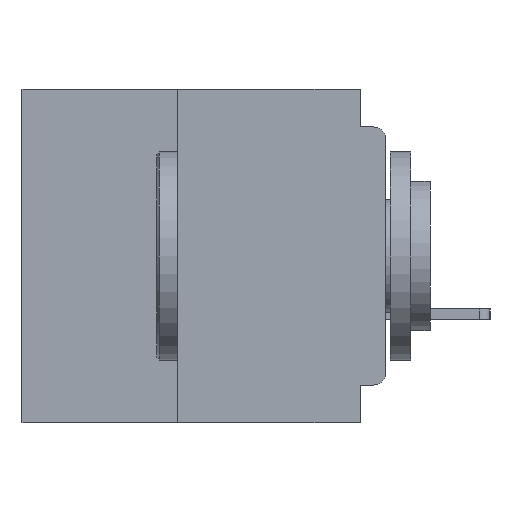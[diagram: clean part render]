
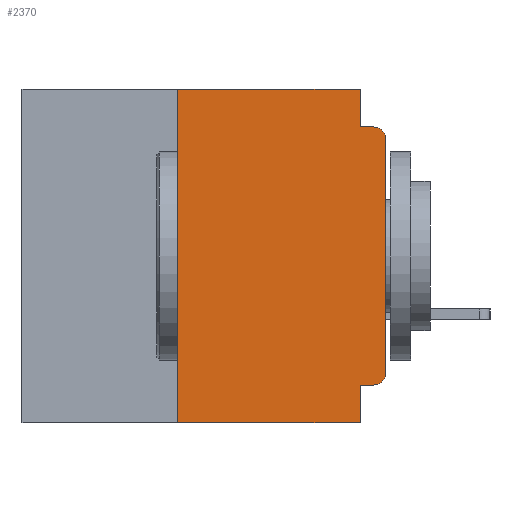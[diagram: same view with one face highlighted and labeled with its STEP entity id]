
A CAD part, left-side view. The second image highlights one B-rep face of the part: STEP entity #2370.
In plain terms, the highlighted planar face has unit normal (-1, 0, 0).
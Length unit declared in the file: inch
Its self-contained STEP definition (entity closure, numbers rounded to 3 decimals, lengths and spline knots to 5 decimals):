
#1368 = VECTOR ( 'NONE', #28148, 39.37008 ) ;
#1810 = VERTEX_POINT ( 'NONE', #24795 ) ;
#2370 = ADVANCED_FACE ( 'NONE', ( #47986 ), #18815, .F. ) ;
#2901 = EDGE_CURVE ( 'NONE', #58444, #57417, #28185, .T. ) ;
#2973 = LINE ( 'NONE', #21634, #39948 ) ;
#4911 = EDGE_CURVE ( 'NONE', #58444, #41368, #53182, .T. ) ;
#6284 = DIRECTION ( 'NONE',  ( 0., 0., -1. ) ) ;
#6732 = DIRECTION ( 'NONE',  ( 0., 0., -1. ) ) ;
#7279 = ORIENTED_EDGE ( 'NONE', *, *, #32563, .F. ) ;
#7483 = VECTOR ( 'NONE', #6284, 39.37008 ) ;
#8209 = CARTESIAN_POINT ( 'NONE',  ( 0., 0.015, -0.34 ) ) ;
#9074 = LINE ( 'NONE', #31262, #7483 ) ;
#9985 = EDGE_CURVE ( 'NONE', #29424, #62762, #27949, .T. ) ;
#13242 = DIRECTION ( 'NONE',  ( 0., 0., -1. ) ) ;
#13811 = CARTESIAN_POINT ( 'NONE',  ( 0., 0.437, 0. ) ) ;
#14759 = ORIENTED_EDGE ( 'NONE', *, *, #9985, .T. ) ;
#15155 = CARTESIAN_POINT ( 'NONE',  ( 0., 0.031, -0.4 ) ) ;
#15238 = CARTESIAN_POINT ( 'NONE',  ( 0., 0.015, -0.045 ) ) ;
#16145 = CARTESIAN_POINT ( 'NONE',  ( 0., 0., 0. ) ) ;
#16833 = CARTESIAN_POINT ( 'NONE',  ( 0., 0.437, 0. ) ) ;
#17778 = ORIENTED_EDGE ( 'NONE', *, *, #55778, .F. ) ;
#18815 = PLANE ( 'NONE',  #31830 ) ;
#20260 = AXIS2_PLACEMENT_3D ( 'NONE', #23625, #58712, #28629 ) ;
#21634 = CARTESIAN_POINT ( 'NONE',  ( 0., 0.031, -0.4 ) ) ;
#22276 = ORIENTED_EDGE ( 'NONE', *, *, #56730, .F. ) ;
#23041 = ORIENTED_EDGE ( 'NONE', *, *, #2901, .T. ) ;
#23466 = ORIENTED_EDGE ( 'NONE', *, *, #38846, .F. ) ;
#23625 = CARTESIAN_POINT ( 'NONE',  ( 0., 0.015, -0.06 ) ) ;
#23858 = DIRECTION ( 'NONE',  ( 0., 0., -1. ) ) ;
#24396 = VERTEX_POINT ( 'NONE', #15238 ) ;
#24795 = CARTESIAN_POINT ( 'NONE',  ( 0., 0., -0.06 ) ) ;
#25496 = CARTESIAN_POINT ( 'NONE',  ( 0., 0.031, 0. ) ) ;
#25714 = CARTESIAN_POINT ( 'NONE',  ( 0., 0.25, -0.4 ) ) ;
#25757 = EDGE_LOOP ( 'NONE', ( #57913, #36487, #22276, #33500, #23466, #64864, #23041, #7279, #17778, #14759 ) ) ;
#25986 = LINE ( 'NONE', #56144, #29111 ) ;
#27949 = CIRCLE ( 'NONE', #29589, 0.015 ) ;
#27997 = CIRCLE ( 'NONE', #20260, 0.015 ) ;
#28148 = DIRECTION ( 'NONE',  ( 0., -1., 0. ) ) ;
#28185 = LINE ( 'NONE', #48216, #1368 ) ;
#28629 = DIRECTION ( 'NONE',  ( 0., 0., -1. ) ) ;
#28829 = EDGE_CURVE ( 'NONE', #1810, #24396, #27997, .T. ) ;
#29111 = VECTOR ( 'NONE', #40977, 39.37008 ) ;
#29424 = VERTEX_POINT ( 'NONE', #57998 ) ;
#29589 = AXIS2_PLACEMENT_3D ( 'NONE', #8209, #43327, #13242 ) ;
#30297 = VECTOR ( 'NONE', #56963, 39.37008 ) ;
#30745 = DIRECTION ( 'NONE',  ( 0., 0., 1. ) ) ;
#30748 = EDGE_CURVE ( 'NONE', #50210, #53123, #9074, .T. ) ;
#31262 = CARTESIAN_POINT ( 'NONE',  ( 0., 0.031, 0. ) ) ;
#31830 = AXIS2_PLACEMENT_3D ( 'NONE', #13811, #38754, #23858 ) ;
#32563 = EDGE_CURVE ( 'NONE', #51239, #57417, #2973, .T. ) ;
#32869 = CARTESIAN_POINT ( 'NONE',  ( 0., 0.25, -0.4 ) ) ;
#33274 = VECTOR ( 'NONE', #56060, 39.37008 ) ;
#33500 = ORIENTED_EDGE ( 'NONE', *, *, #30748, .F. ) ;
#34853 = LINE ( 'NONE', #16145, #33274 ) ;
#36487 = ORIENTED_EDGE ( 'NONE', *, *, #28829, .T. ) ;
#38754 = DIRECTION ( 'NONE',  ( 1., 0., 0. ) ) ;
#38846 = EDGE_CURVE ( 'NONE', #41368, #50210, #57040, .T. ) ;
#38948 = CARTESIAN_POINT ( 'NONE',  ( 0., 0.031, -0.355 ) ) ;
#39948 = VECTOR ( 'NONE', #6732, 39.37008 ) ;
#40128 = CARTESIAN_POINT ( 'NONE',  ( 0., 0.031, -0.045 ) ) ;
#40977 = DIRECTION ( 'NONE',  ( 0., 1., 0. ) ) ;
#41368 = VERTEX_POINT ( 'NONE', #53995 ) ;
#43327 = DIRECTION ( 'NONE',  ( -1., 0., 0. ) ) ;
#44426 = DIRECTION ( 'NONE',  ( 0., -1., 0. ) ) ;
#47915 = VECTOR ( 'NONE', #44426, 39.37008 ) ;
#47986 = FACE_OUTER_BOUND ( 'NONE', #25757, .T. ) ;
#48216 = CARTESIAN_POINT ( 'NONE',  ( 0., 0.437, -0.4 ) ) ;
#49495 = LINE ( 'NONE', #64295, #47915 ) ;
#50210 = VERTEX_POINT ( 'NONE', #25496 ) ;
#50608 = CARTESIAN_POINT ( 'NONE',  ( 0., 0., -0.34 ) ) ;
#51239 = VERTEX_POINT ( 'NONE', #38948 ) ;
#53123 = VERTEX_POINT ( 'NONE', #40128 ) ;
#53182 = LINE ( 'NONE', #25714, #54759 ) ;
#53995 = CARTESIAN_POINT ( 'NONE',  ( 0., 0.25, 0. ) ) ;
#54759 = VECTOR ( 'NONE', #30745, 39.37008 ) ;
#55778 = EDGE_CURVE ( 'NONE', #29424, #51239, #25986, .T. ) ;
#56060 = DIRECTION ( 'NONE',  ( 0., 0., 1. ) ) ;
#56144 = CARTESIAN_POINT ( 'NONE',  ( 0., 0., -0.355 ) ) ;
#56730 = EDGE_CURVE ( 'NONE', #53123, #24396, #49495, .T. ) ;
#56963 = DIRECTION ( 'NONE',  ( 0., -1., 0. ) ) ;
#57040 = LINE ( 'NONE', #16833, #30297 ) ;
#57417 = VERTEX_POINT ( 'NONE', #15155 ) ;
#57913 = ORIENTED_EDGE ( 'NONE', *, *, #59456, .T. ) ;
#57998 = CARTESIAN_POINT ( 'NONE',  ( 0., 0.015, -0.355 ) ) ;
#58444 = VERTEX_POINT ( 'NONE', #32869 ) ;
#58712 = DIRECTION ( 'NONE',  ( -1., 0., 0. ) ) ;
#59456 = EDGE_CURVE ( 'NONE', #62762, #1810, #34853, .T. ) ;
#62762 = VERTEX_POINT ( 'NONE', #50608 ) ;
#64295 = CARTESIAN_POINT ( 'NONE',  ( 0., 0., -0.045 ) ) ;
#64864 = ORIENTED_EDGE ( 'NONE', *, *, #4911, .F. ) ;
